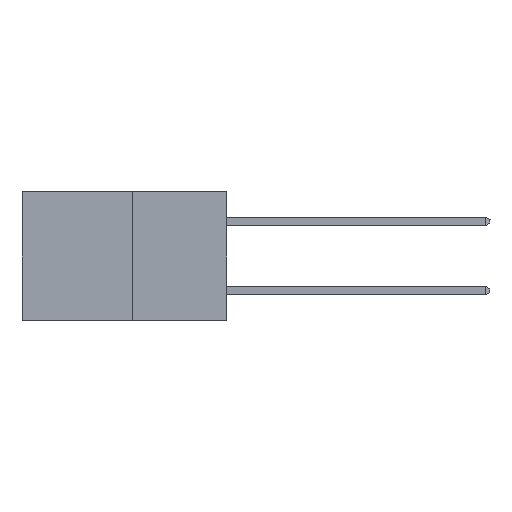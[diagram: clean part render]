
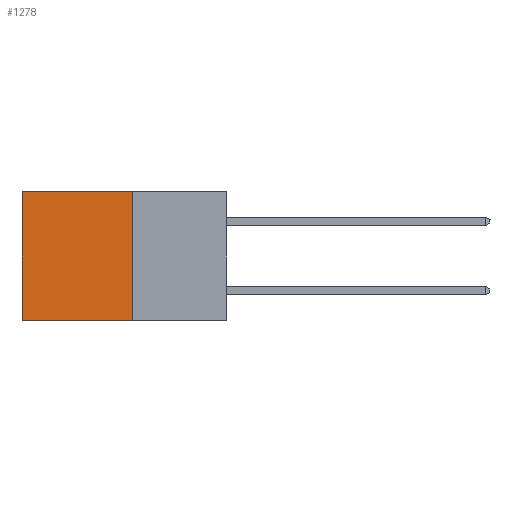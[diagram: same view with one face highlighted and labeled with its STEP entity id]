
A CAD part, left-side view. The second image highlights one B-rep face of the part: STEP entity #1278.
In plain terms, the highlighted planar face has unit normal (-1, 0, 0).
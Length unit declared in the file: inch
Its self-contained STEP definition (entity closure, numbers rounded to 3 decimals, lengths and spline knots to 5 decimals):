
#194 = EDGE_CURVE ( 'NONE', #7906, #1533, #7942, .T. ) ;
#361 = ORIENTED_EDGE ( 'NONE', *, *, #17273, .T. ) ;
#1278 = ADVANCED_FACE ( 'NONE', ( #16028 ), #10782, .F. ) ;
#1533 = VERTEX_POINT ( 'NONE', #16813 ) ;
#2765 = VECTOR ( 'NONE', #11015, 39.37008 ) ;
#2833 = CARTESIAN_POINT ( 'NONE',  ( 0.277, 0.27, -0.37 ) ) ;
#3830 = CARTESIAN_POINT ( 'NONE',  ( 0.277, 0.27, -0.37 ) ) ;
#4314 = VECTOR ( 'NONE', #15136, 39.37008 ) ;
#4809 = CARTESIAN_POINT ( 'NONE',  ( 0.277, 0.27, 0. ) ) ;
#5091 = DIRECTION ( 'NONE',  ( 0., 0., -1. ) ) ;
#5818 = ORIENTED_EDGE ( 'NONE', *, *, #194, .T. ) ;
#5859 = CARTESIAN_POINT ( 'NONE',  ( 0.277, 0.27, -0.37 ) ) ;
#6114 = CARTESIAN_POINT ( 'NONE',  ( 0.277, 0.27, -0.37 ) ) ;
#6120 = CARTESIAN_POINT ( 'NONE',  ( 0.277, 0.59, -0.37 ) ) ;
#6624 = ORIENTED_EDGE ( 'NONE', *, *, #9291, .F. ) ;
#6820 = LINE ( 'NONE', #2833, #2765 ) ;
#7063 = VERTEX_POINT ( 'NONE', #6120 ) ;
#7344 = EDGE_CURVE ( 'NONE', #14023, #7063, #6820, .T. ) ;
#7463 = ORIENTED_EDGE ( 'NONE', *, *, #7344, .F. ) ;
#7906 = VERTEX_POINT ( 'NONE', #4809 ) ;
#7942 = LINE ( 'NONE', #8652, #4314 ) ;
#8023 = LINE ( 'NONE', #11885, #15113 ) ;
#8652 = CARTESIAN_POINT ( 'NONE',  ( 0.277, 0.27, 0. ) ) ;
#9291 = EDGE_CURVE ( 'NONE', #7906, #14023, #10417, .T. ) ;
#9317 = DIRECTION ( 'NONE',  ( 1., 0., 0. ) ) ;
#10043 = AXIS2_PLACEMENT_3D ( 'NONE', #5859, #9317, #10843 ) ;
#10417 = LINE ( 'NONE', #6114, #16974 ) ;
#10782 = PLANE ( 'NONE',  #10043 ) ;
#10843 = DIRECTION ( 'NONE',  ( 0., 0., -1. ) ) ;
#11015 = DIRECTION ( 'NONE',  ( 0., 1., 0. ) ) ;
#11494 = EDGE_LOOP ( 'NONE', ( #361, #7463, #6624, #5818 ) ) ;
#11885 = CARTESIAN_POINT ( 'NONE',  ( 0.277, 0.59, -0.37 ) ) ;
#14023 = VERTEX_POINT ( 'NONE', #3830 ) ;
#14189 = DIRECTION ( 'NONE',  ( 0., 0., -1. ) ) ;
#15113 = VECTOR ( 'NONE', #5091, 39.37008 ) ;
#15136 = DIRECTION ( 'NONE',  ( 0., 1., 0. ) ) ;
#16028 = FACE_OUTER_BOUND ( 'NONE', #11494, .T. ) ;
#16813 = CARTESIAN_POINT ( 'NONE',  ( 0.277, 0.59, 0. ) ) ;
#16974 = VECTOR ( 'NONE', #14189, 39.37008 ) ;
#17273 = EDGE_CURVE ( 'NONE', #1533, #7063, #8023, .T. ) ;
